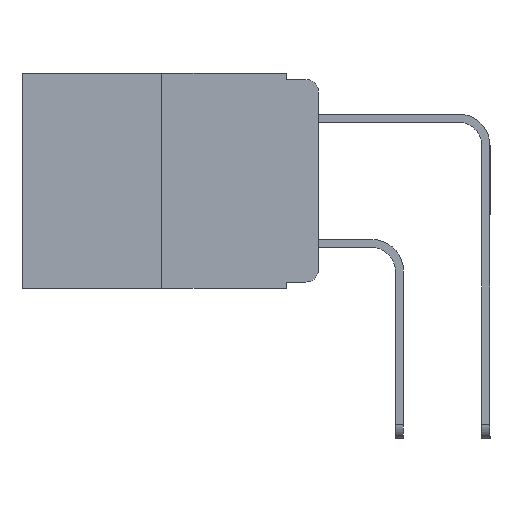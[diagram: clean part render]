
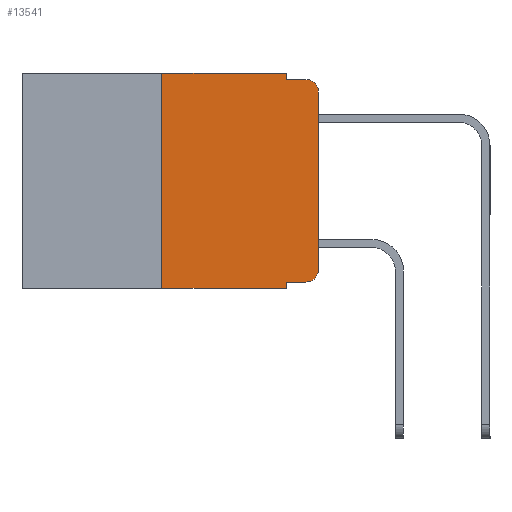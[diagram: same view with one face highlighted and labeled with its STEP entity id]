
A CAD part, left-side view. The second image highlights one B-rep face of the part: STEP entity #13541.
In plain terms, the highlighted planar face has unit normal (-1, 0, 0).
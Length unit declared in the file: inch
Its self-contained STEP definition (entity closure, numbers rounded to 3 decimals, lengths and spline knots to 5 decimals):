
#336 = CARTESIAN_POINT ( 'NONE',  ( 0., 0., -0.03 ) ) ;
#1261 = DIRECTION ( 'NONE',  ( 0., -1., 0. ) ) ;
#1304 = VERTEX_POINT ( 'NONE', #16486 ) ;
#1599 = DIRECTION ( 'NONE',  ( 0., 0., 1. ) ) ;
#1912 = ORIENTED_EDGE ( 'NONE', *, *, #13620, .F. ) ;
#2049 = AXIS2_PLACEMENT_3D ( 'NONE', #14725, #6045, #16192 ) ;
#2276 = VECTOR ( 'NONE', #10524, 39.37008 ) ;
#2359 = CARTESIAN_POINT ( 'NONE',  ( 0., 0.051, 0. ) ) ;
#2547 = VERTEX_POINT ( 'NONE', #11029 ) ;
#2884 = PLANE ( 'NONE',  #9281 ) ;
#3010 = CARTESIAN_POINT ( 'NONE',  ( 0., 0.25, 0. ) ) ;
#3055 = CARTESIAN_POINT ( 'NONE',  ( 0., 0.02, -0.03 ) ) ;
#3354 = ORIENTED_EDGE ( 'NONE', *, *, #11688, .F. ) ;
#3487 = VERTEX_POINT ( 'NONE', #15094 ) ;
#3890 = DIRECTION ( 'NONE',  ( 0., 0., -1. ) ) ;
#4221 = VECTOR ( 'NONE', #4530, 39.37008 ) ;
#4249 = CARTESIAN_POINT ( 'NONE',  ( 0., 0.051, -0.333 ) ) ;
#4530 = DIRECTION ( 'NONE',  ( 0., 0., 1. ) ) ;
#4577 = DIRECTION ( 'NONE',  ( 0., 0., -1. ) ) ;
#4685 = FACE_OUTER_BOUND ( 'NONE', #4821, .T. ) ;
#4821 = EDGE_LOOP ( 'NONE', ( #15713, #12707, #16600, #1912, #5955, #9795, #17902, #3354, #15051, #15487 ) ) ;
#5173 = CARTESIAN_POINT ( 'NONE',  ( 0., 0.473, -0.343 ) ) ;
#5639 = VECTOR ( 'NONE', #1261, 39.37008 ) ;
#5647 = DIRECTION ( 'NONE',  ( 0., -1., 0. ) ) ;
#5955 = ORIENTED_EDGE ( 'NONE', *, *, #13501, .F. ) ;
#5964 = DIRECTION ( 'NONE',  ( 0., 0., -1. ) ) ;
#6045 = DIRECTION ( 'NONE',  ( -1., 0., 0. ) ) ;
#6118 = CARTESIAN_POINT ( 'NONE',  ( 0., 0., 0. ) ) ;
#6134 = LINE ( 'NONE', #14506, #5639 ) ;
#6754 = AXIS2_PLACEMENT_3D ( 'NONE', #3055, #13292, #4577 ) ;
#7091 = VECTOR ( 'NONE', #1599, 39.37008 ) ;
#7232 = VERTEX_POINT ( 'NONE', #18449 ) ;
#7262 = VERTEX_POINT ( 'NONE', #9929 ) ;
#8247 = VECTOR ( 'NONE', #3890, 39.37008 ) ;
#8556 = VERTEX_POINT ( 'NONE', #8945 ) ;
#8945 = CARTESIAN_POINT ( 'NONE',  ( 0., 0.051, 0. ) ) ;
#9083 = CARTESIAN_POINT ( 'NONE',  ( 0., 0.051, 0. ) ) ;
#9281 = AXIS2_PLACEMENT_3D ( 'NONE', #13140, #14654, #5964 ) ;
#9730 = EDGE_CURVE ( 'NONE', #7262, #17573, #18300, .T. ) ;
#9795 = ORIENTED_EDGE ( 'NONE', *, *, #12609, .F. ) ;
#9880 = CARTESIAN_POINT ( 'NONE',  ( 0., 0.051, -0.343 ) ) ;
#9929 = CARTESIAN_POINT ( 'NONE',  ( 0., 0.02, -0.333 ) ) ;
#10052 = CARTESIAN_POINT ( 'NONE',  ( 0., 0., -0.313 ) ) ;
#10262 = LINE ( 'NONE', #5173, #17916 ) ;
#10524 = DIRECTION ( 'NONE',  ( 0., 0., -1. ) ) ;
#10729 = EDGE_CURVE ( 'NONE', #11905, #7262, #14751, .T. ) ;
#10917 = LINE ( 'NONE', #6118, #7091 ) ;
#11029 = CARTESIAN_POINT ( 'NONE',  ( 0., 0.25, 0. ) ) ;
#11428 = CARTESIAN_POINT ( 'NONE',  ( 0., 0.051, -0.01 ) ) ;
#11688 = EDGE_CURVE ( 'NONE', #11905, #15997, #15963, .T. ) ;
#11905 = VERTEX_POINT ( 'NONE', #18865 ) ;
#12096 = CIRCLE ( 'NONE', #6754, 0.02 ) ;
#12609 = EDGE_CURVE ( 'NONE', #7232, #2547, #16366, .T. ) ;
#12707 = ORIENTED_EDGE ( 'NONE', *, *, #15587, .T. ) ;
#13140 = CARTESIAN_POINT ( 'NONE',  ( 0., 0.473, 0. ) ) ;
#13292 = DIRECTION ( 'NONE',  ( -1., 0., 0. ) ) ;
#13501 = EDGE_CURVE ( 'NONE', #2547, #8556, #6134, .T. ) ;
#13541 = ADVANCED_FACE ( 'NONE', ( #4685 ), #2884, .F. ) ;
#13620 = EDGE_CURVE ( 'NONE', #8556, #3487, #14974, .T. ) ;
#14137 = VECTOR ( 'NONE', #5647, 39.37008 ) ;
#14506 = CARTESIAN_POINT ( 'NONE',  ( 0., 0.473, 0. ) ) ;
#14611 = EDGE_CURVE ( 'NONE', #3487, #1304, #17943, .T. ) ;
#14654 = DIRECTION ( 'NONE',  ( 1., 0., 0. ) ) ;
#14725 = CARTESIAN_POINT ( 'NONE',  ( 0., 0.02, -0.313 ) ) ;
#14751 = LINE ( 'NONE', #4249, #18054 ) ;
#14974 = LINE ( 'NONE', #9083, #2276 ) ;
#15051 = ORIENTED_EDGE ( 'NONE', *, *, #10729, .T. ) ;
#15094 = CARTESIAN_POINT ( 'NONE',  ( 0., 0.051, -0.01 ) ) ;
#15487 = ORIENTED_EDGE ( 'NONE', *, *, #9730, .T. ) ;
#15587 = EDGE_CURVE ( 'NONE', #16649, #1304, #12096, .T. ) ;
#15713 = ORIENTED_EDGE ( 'NONE', *, *, #16544, .T. ) ;
#15963 = LINE ( 'NONE', #2359, #8247 ) ;
#15981 = DIRECTION ( 'NONE',  ( 0., -1., 0. ) ) ;
#15997 = VERTEX_POINT ( 'NONE', #9880 ) ;
#16192 = DIRECTION ( 'NONE',  ( 0., 0., -1. ) ) ;
#16366 = LINE ( 'NONE', #3010, #4221 ) ;
#16486 = CARTESIAN_POINT ( 'NONE',  ( 0., 0.02, -0.01 ) ) ;
#16544 = EDGE_CURVE ( 'NONE', #17573, #16649, #10917, .T. ) ;
#16600 = ORIENTED_EDGE ( 'NONE', *, *, #14611, .F. ) ;
#16649 = VERTEX_POINT ( 'NONE', #336 ) ;
#16792 = DIRECTION ( 'NONE',  ( 0., -1., 0. ) ) ;
#17573 = VERTEX_POINT ( 'NONE', #10052 ) ;
#17902 = ORIENTED_EDGE ( 'NONE', *, *, #18042, .T. ) ;
#17916 = VECTOR ( 'NONE', #16792, 39.37008 ) ;
#17943 = LINE ( 'NONE', #11428, #14137 ) ;
#18042 = EDGE_CURVE ( 'NONE', #7232, #15997, #10262, .T. ) ;
#18054 = VECTOR ( 'NONE', #15981, 39.37008 ) ;
#18300 = CIRCLE ( 'NONE', #2049, 0.02 ) ;
#18449 = CARTESIAN_POINT ( 'NONE',  ( 0., 0.25, -0.343 ) ) ;
#18865 = CARTESIAN_POINT ( 'NONE',  ( 0., 0.051, -0.333 ) ) ;
